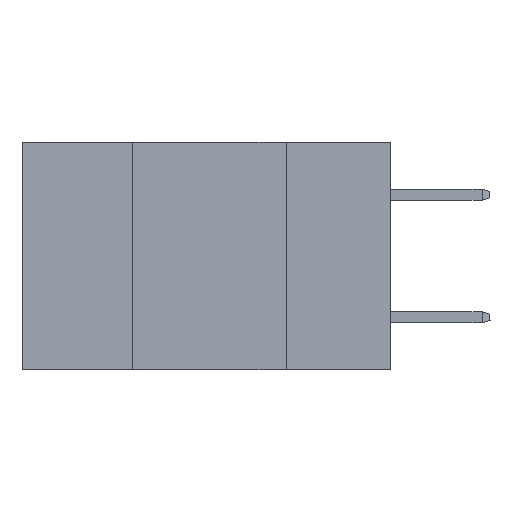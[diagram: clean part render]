
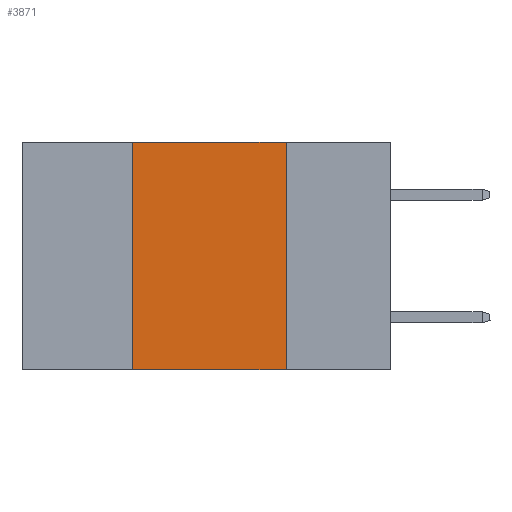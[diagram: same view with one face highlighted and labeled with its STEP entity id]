
A CAD part, left-side view. The second image highlights one B-rep face of the part: STEP entity #3871.
In plain terms, the highlighted planar face has unit normal (-1, 0, 0).
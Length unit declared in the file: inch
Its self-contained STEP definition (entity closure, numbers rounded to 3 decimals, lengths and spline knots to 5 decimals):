
#300 = DIRECTION ( 'NONE',  ( 0., -1., 0. ) ) ;
#1872 = AXIS2_PLACEMENT_3D ( 'NONE', #27602, #5144, #24558 ) ;
#2040 = VERTEX_POINT ( 'NONE', #11274 ) ;
#2810 = PLANE ( 'NONE',  #1872 ) ;
#3468 = VECTOR ( 'NONE', #16252, 39.37008 ) ;
#3871 = ADVANCED_FACE ( 'NONE', ( #8557 ), #2810, .F. ) ;
#4304 = ORIENTED_EDGE ( 'NONE', *, *, #34198, .F. ) ;
#5144 = DIRECTION ( 'NONE',  ( 1., 0., 0. ) ) ;
#6292 = VERTEX_POINT ( 'NONE', #8482 ) ;
#6379 = ORIENTED_EDGE ( 'NONE', *, *, #18290, .F. ) ;
#7629 = EDGE_CURVE ( 'NONE', #2040, #26417, #10491, .T. ) ;
#8482 = CARTESIAN_POINT ( 'NONE',  ( 0., 0.42, 0. ) ) ;
#8557 = FACE_OUTER_BOUND ( 'NONE', #12020, .T. ) ;
#9273 = LINE ( 'NONE', #9445, #10462 ) ;
#9445 = CARTESIAN_POINT ( 'NONE',  ( 0., 0.6, -0.37 ) ) ;
#9618 = DIRECTION ( 'NONE',  ( 0., -1., 0. ) ) ;
#10462 = VECTOR ( 'NONE', #9618, 39.37008 ) ;
#10491 = LINE ( 'NONE', #12649, #3468 ) ;
#11274 = CARTESIAN_POINT ( 'NONE',  ( 0., 0.17, 0. ) ) ;
#12020 = EDGE_LOOP ( 'NONE', ( #27777, #6379, #4304, #29890 ) ) ;
#12649 = CARTESIAN_POINT ( 'NONE',  ( 0., 0.17, 0. ) ) ;
#13978 = LINE ( 'NONE', #22256, #34247 ) ;
#16252 = DIRECTION ( 'NONE',  ( 0., 0., -1. ) ) ;
#18290 = EDGE_CURVE ( 'NONE', #6292, #2040, #13978, .T. ) ;
#19066 = CARTESIAN_POINT ( 'NONE',  ( 0., 0.17, -0.37 ) ) ;
#20991 = CARTESIAN_POINT ( 'NONE',  ( 0., 0.42, -0.37 ) ) ;
#22256 = CARTESIAN_POINT ( 'NONE',  ( 0., 0.6, 0. ) ) ;
#23789 = EDGE_CURVE ( 'NONE', #32934, #26417, #9273, .T. ) ;
#24558 = DIRECTION ( 'NONE',  ( 0., 0., -1. ) ) ;
#26417 = VERTEX_POINT ( 'NONE', #19066 ) ;
#27602 = CARTESIAN_POINT ( 'NONE',  ( 0., 0.6, 0. ) ) ;
#27777 = ORIENTED_EDGE ( 'NONE', *, *, #7629, .F. ) ;
#28032 = CARTESIAN_POINT ( 'NONE',  ( 0., 0.42, 0. ) ) ;
#28200 = DIRECTION ( 'NONE',  ( 0., 0., 1. ) ) ;
#29890 = ORIENTED_EDGE ( 'NONE', *, *, #23789, .T. ) ;
#30378 = LINE ( 'NONE', #28032, #34210 ) ;
#32934 = VERTEX_POINT ( 'NONE', #20991 ) ;
#34198 = EDGE_CURVE ( 'NONE', #32934, #6292, #30378, .T. ) ;
#34210 = VECTOR ( 'NONE', #28200, 39.37008 ) ;
#34247 = VECTOR ( 'NONE', #300, 39.37008 ) ;
